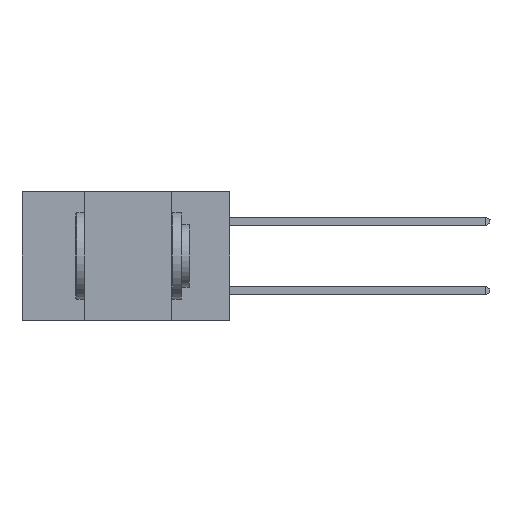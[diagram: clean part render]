
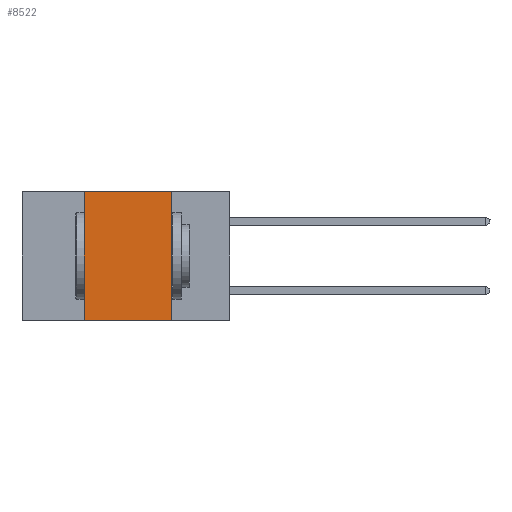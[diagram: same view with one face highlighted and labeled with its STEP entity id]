
A CAD part, left-side view. The second image highlights one B-rep face of the part: STEP entity #8522.
In plain terms, the highlighted planar face has unit normal (-1, 0, 0).
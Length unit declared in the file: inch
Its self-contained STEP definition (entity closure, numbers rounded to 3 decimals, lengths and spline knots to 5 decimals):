
#1600 = VECTOR ( 'NONE', #5954, 39.37008 ) ;
#1917 = PLANE ( 'NONE',  #2837 ) ;
#2225 = EDGE_CURVE ( 'NONE', #14682, #6232, #18771, .T. ) ;
#2837 = AXIS2_PLACEMENT_3D ( 'NONE', #9208, #16928, #10969 ) ;
#3002 = FACE_OUTER_BOUND ( 'NONE', #14066, .T. ) ;
#4074 = CARTESIAN_POINT ( 'NONE',  ( 0., 0.42, 0. ) ) ;
#5954 = DIRECTION ( 'NONE',  ( 0., 0., -1. ) ) ;
#6206 = EDGE_CURVE ( 'NONE', #19002, #6232, #7553, .T. ) ;
#6232 = VERTEX_POINT ( 'NONE', #12198 ) ;
#6407 = DIRECTION ( 'NONE',  ( 0., 0., 1. ) ) ;
#7455 = CARTESIAN_POINT ( 'NONE',  ( 0., 0.17, -0.37 ) ) ;
#7553 = LINE ( 'NONE', #7455, #1600 ) ;
#8522 = ADVANCED_FACE ( 'NONE', ( #3002 ), #1917, .F. ) ;
#8567 = EDGE_CURVE ( 'NONE', #14682, #14845, #15534, .T. ) ;
#9195 = VECTOR ( 'NONE', #17173, 39.37008 ) ;
#9208 = CARTESIAN_POINT ( 'NONE',  ( 0., 0.6, 0. ) ) ;
#10600 = LINE ( 'NONE', #15060, #11822 ) ;
#10602 = CARTESIAN_POINT ( 'NONE',  ( 0., 0.17, 0. ) ) ;
#10783 = VECTOR ( 'NONE', #6407, 39.37008 ) ;
#10969 = DIRECTION ( 'NONE',  ( 0., 0., -1. ) ) ;
#11110 = CARTESIAN_POINT ( 'NONE',  ( 0., 0.6, -0.37 ) ) ;
#11477 = ORIENTED_EDGE ( 'NONE', *, *, #8567, .F. ) ;
#11506 = ORIENTED_EDGE ( 'NONE', *, *, #2225, .T. ) ;
#11822 = VECTOR ( 'NONE', #14877, 39.37008 ) ;
#12198 = CARTESIAN_POINT ( 'NONE',  ( 0., 0.17, -0.37 ) ) ;
#12968 = ORIENTED_EDGE ( 'NONE', *, *, #6206, .F. ) ;
#14066 = EDGE_LOOP ( 'NONE', ( #12968, #18447, #11477, #11506 ) ) ;
#14682 = VERTEX_POINT ( 'NONE', #18505 ) ;
#14845 = VERTEX_POINT ( 'NONE', #4074 ) ;
#14877 = DIRECTION ( 'NONE',  ( 0., -1., 0. ) ) ;
#15060 = CARTESIAN_POINT ( 'NONE',  ( 0., 0.6, 0. ) ) ;
#15534 = LINE ( 'NONE', #18438, #10783 ) ;
#16718 = EDGE_CURVE ( 'NONE', #14845, #19002, #10600, .T. ) ;
#16928 = DIRECTION ( 'NONE',  ( 1., 0., 0. ) ) ;
#17173 = DIRECTION ( 'NONE',  ( 0., -1., 0. ) ) ;
#18438 = CARTESIAN_POINT ( 'NONE',  ( 0., 0.42, -0.37 ) ) ;
#18447 = ORIENTED_EDGE ( 'NONE', *, *, #16718, .F. ) ;
#18505 = CARTESIAN_POINT ( 'NONE',  ( 0., 0.42, -0.37 ) ) ;
#18771 = LINE ( 'NONE', #11110, #9195 ) ;
#19002 = VERTEX_POINT ( 'NONE', #10602 ) ;
